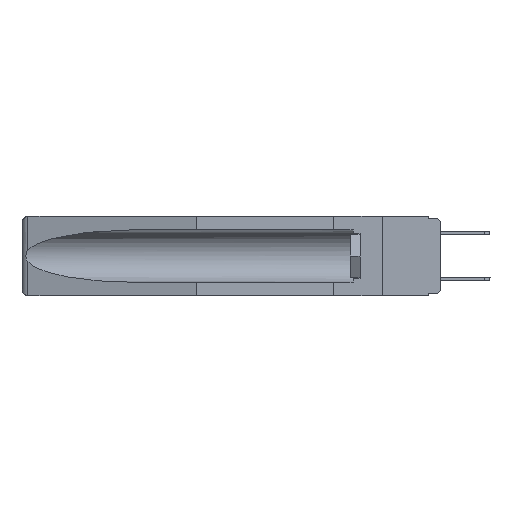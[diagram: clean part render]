
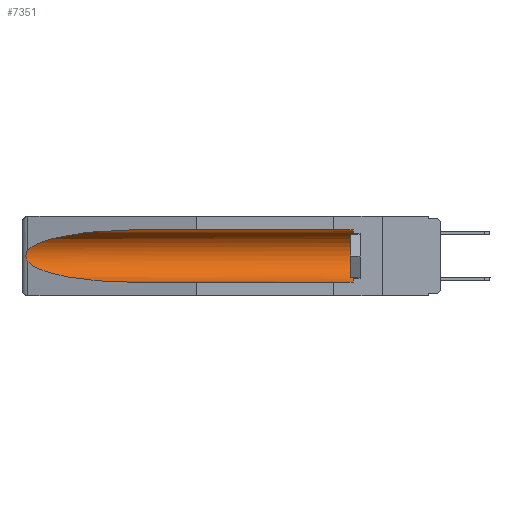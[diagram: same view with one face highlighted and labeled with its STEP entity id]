
A CAD part, left-side view. The second image highlights one B-rep face of the part: STEP entity #7351.
In plain terms, the highlighted cylindrical face has radius 2.857 mm (diameter 5.715 mm), a partial arc.
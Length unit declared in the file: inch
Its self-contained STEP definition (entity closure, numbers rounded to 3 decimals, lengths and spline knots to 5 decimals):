
#375 =( BOUNDED_CURVE ( )  B_SPLINE_CURVE ( 3, ( #3941, #9322, #17759, #12080 ),
 .UNSPECIFIED., .F., .F. ) 
 B_SPLINE_CURVE_WITH_KNOTS ( ( 4, 4 ),
 ( 0.1948, 1.5708 ),
 .UNSPECIFIED. ) 
 CURVE ( )  GEOMETRIC_REPRESENTATION_ITEM ( )  RATIONAL_B_SPLINE_CURVE ( ( 1., 0.848, 0.848, 1. ) ) 
 REPRESENTATION_ITEM ( '' )  );
#1135 = CARTESIAN_POINT ( 'NONE',  ( 0.2675, 1.53308, -0.17534 ) ) ;
#1472 = CARTESIAN_POINT ( 'NONE',  ( 0.26537, 1.52718, -0.14972 ) ) ;
#1668 = VECTOR ( 'NONE', #1705, 39.37008 ) ;
#1705 = DIRECTION ( 'NONE',  ( 0., 1., 0. ) ) ;
#1807 = FACE_OUTER_BOUND ( 'NONE', #4847, .T. ) ;
#2086 = CARTESIAN_POINT ( 'NONE',  ( 0.26654, 1.53092, -0.15636 ) ) ;
#2326 = VERTEX_POINT ( 'NONE', #8978 ) ;
#2890 = CIRCLE ( 'NONE', #7620, 0.1125 ) ;
#2932 = DIRECTION ( 'NONE',  ( 0., 1., 0. ) ) ;
#2956 = ORIENTED_EDGE ( 'NONE', *, *, #12872, .T. ) ;
#2963 = CARTESIAN_POINT ( 'NONE',  ( 0.155, 1.07973, -0.059 ) ) ;
#3081 = CARTESIAN_POINT ( 'NONE',  ( 0.155, 1.07973, -0.059 ) ) ;
#3567 = ORIENTED_EDGE ( 'NONE', *, *, #9200, .T. ) ;
#3574 = CARTESIAN_POINT ( 'NONE',  ( 0.2673, 1.5327, -0.16383 ) ) ;
#3941 = CARTESIAN_POINT ( 'NONE',  ( 0.26537, 1.52718, -0.19328 ) ) ;
#4108 = CARTESIAN_POINT ( 'NONE',  ( 0.26597, 1.5296, -0.19026 ) ) ;
#4847 = EDGE_LOOP ( 'NONE', ( #7223, #2956, #16475, #11851, #3567, #12553 ) ) ;
#5218 = CARTESIAN_POINT ( 'NONE',  ( 0.2673, 1.53269, -0.17917 ) ) ;
#5453 = DIRECTION ( 'NONE',  ( 0., -1., 0. ) ) ;
#5794 = CARTESIAN_POINT ( 'NONE',  ( 0.155, -0.30754, -0.059 ) ) ;
#6286 = VERTEX_POINT ( 'NONE', #8072 ) ;
#6895 = B_SPLINE_CURVE_WITH_KNOTS ( 'NONE', 3,
 ( #17355, #13256, #2086, #3574, #14939, #1135, #5218, #16757, #4108, #13890 ),
 .UNSPECIFIED., .F., .F.,
 ( 4, 2, 2, 2, 4 ),
 ( 0., 0.00029, 0.00058, 0.00087, 0.00117 ),
 .UNSPECIFIED. ) ;
#7223 = ORIENTED_EDGE ( 'NONE', *, *, #10641, .T. ) ;
#7351 = ADVANCED_FACE ( 'NONE', ( #1807 ), #8632, .F. ) ;
#7577 = CARTESIAN_POINT ( 'NONE',  ( 0.26537, 1.52718, -0.14972 ) ) ;
#7620 = AXIS2_PLACEMENT_3D ( 'NONE', #9515, #5453, #16370 ) ;
#8072 = CARTESIAN_POINT ( 'NONE',  ( 0.155, 1.07973, -0.284 ) ) ;
#8330 = EDGE_CURVE ( 'NONE', #2326, #6286, #375, .T. ) ;
#8632 = CYLINDRICAL_SURFACE ( 'NONE', #14990, 0.1125 ) ;
#8886 = VERTEX_POINT ( 'NONE', #10176 ) ;
#8978 = CARTESIAN_POINT ( 'NONE',  ( 0.26537, 1.52718, -0.19328 ) ) ;
#9200 = EDGE_CURVE ( 'NONE', #14385, #8886, #2890, .T. ) ;
#9322 = CARTESIAN_POINT ( 'NONE',  ( 0.25451, 1.48313, -0.24835 ) ) ;
#9515 = CARTESIAN_POINT ( 'NONE',  ( 0.155, 0.126, -0.1715 ) ) ;
#9788 = CARTESIAN_POINT ( 'NONE',  ( 0.25451, 1.48313, -0.09465 ) ) ;
#9844 = DIRECTION ( 'NONE',  ( 0., 0., 1. ) ) ;
#9945 = LINE ( 'NONE', #5794, #15493 ) ;
#10040 = CARTESIAN_POINT ( 'NONE',  ( 0.155, -0.30754, -0.1715 ) ) ;
#10176 = CARTESIAN_POINT ( 'NONE',  ( 0.155, 0.126, -0.059 ) ) ;
#10641 = EDGE_CURVE ( 'NONE', #13024, #10855, #11235, .T. ) ;
#10855 = VERTEX_POINT ( 'NONE', #7577 ) ;
#11235 =( BOUNDED_CURVE ( )  B_SPLINE_CURVE ( 3, ( #2963, #15443, #9788, #1472 ),
 .UNSPECIFIED., .F., .F. ) 
 B_SPLINE_CURVE_WITH_KNOTS ( ( 4, 4 ),
 ( 4.71239, 6.08839 ),
 .UNSPECIFIED. ) 
 CURVE ( )  GEOMETRIC_REPRESENTATION_ITEM ( )  RATIONAL_B_SPLINE_CURVE ( ( 1., 0.848, 0.848, 1. ) ) 
 REPRESENTATION_ITEM ( '' )  );
#11400 = CARTESIAN_POINT ( 'NONE',  ( 0.155, -0.30754, -0.284 ) ) ;
#11851 = ORIENTED_EDGE ( 'NONE', *, *, #17694, .F. ) ;
#12080 = CARTESIAN_POINT ( 'NONE',  ( 0.155, 1.07973, -0.284 ) ) ;
#12553 = ORIENTED_EDGE ( 'NONE', *, *, #15822, .T. ) ;
#12872 = EDGE_CURVE ( 'NONE', #10855, #2326, #6895, .T. ) ;
#13024 = VERTEX_POINT ( 'NONE', #3081 ) ;
#13256 = CARTESIAN_POINT ( 'NONE',  ( 0.26597, 1.52961, -0.15275 ) ) ;
#13890 = CARTESIAN_POINT ( 'NONE',  ( 0.26537, 1.52718, -0.19328 ) ) ;
#14385 = VERTEX_POINT ( 'NONE', #18275 ) ;
#14939 = CARTESIAN_POINT ( 'NONE',  ( 0.2675, 1.53308, -0.16763 ) ) ;
#14990 = AXIS2_PLACEMENT_3D ( 'NONE', #10040, #15682, #9844 ) ;
#15443 = CARTESIAN_POINT ( 'NONE',  ( 0.21114, 1.30732, -0.059 ) ) ;
#15493 = VECTOR ( 'NONE', #2932, 39.37008 ) ;
#15579 = LINE ( 'NONE', #11400, #1668 ) ;
#15682 = DIRECTION ( 'NONE',  ( 0., 1., 0. ) ) ;
#15822 = EDGE_CURVE ( 'NONE', #8886, #13024, #9945, .T. ) ;
#16370 = DIRECTION ( 'NONE',  ( 0., 0., 1. ) ) ;
#16475 = ORIENTED_EDGE ( 'NONE', *, *, #8330, .T. ) ;
#16757 = CARTESIAN_POINT ( 'NONE',  ( 0.26655, 1.53094, -0.18657 ) ) ;
#17355 = CARTESIAN_POINT ( 'NONE',  ( 0.26537, 1.52718, -0.14972 ) ) ;
#17694 = EDGE_CURVE ( 'NONE', #14385, #6286, #15579, .T. ) ;
#17759 = CARTESIAN_POINT ( 'NONE',  ( 0.21114, 1.30732, -0.284 ) ) ;
#18275 = CARTESIAN_POINT ( 'NONE',  ( 0.155, 0.126, -0.284 ) ) ;
